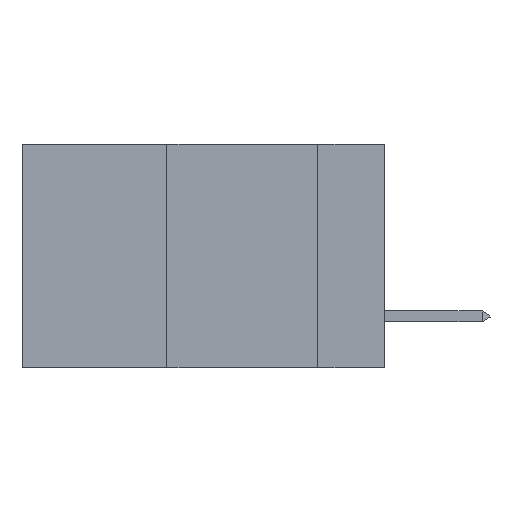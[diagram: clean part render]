
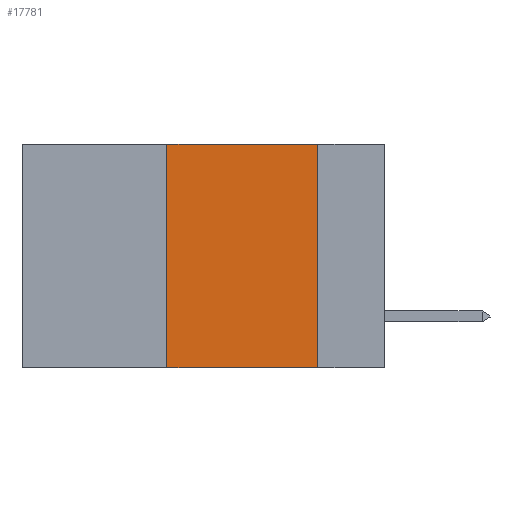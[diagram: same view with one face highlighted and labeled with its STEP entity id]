
A CAD part, left-side view. The second image highlights one B-rep face of the part: STEP entity #17781.
In plain terms, the highlighted planar face has unit normal (-1, 0, 0).
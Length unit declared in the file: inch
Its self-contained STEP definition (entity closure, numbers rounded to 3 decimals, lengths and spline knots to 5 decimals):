
#374 = VERTEX_POINT ( 'NONE', #19010 ) ;
#753 = LINE ( 'NONE', #11042, #24268 ) ;
#932 = EDGE_CURVE ( 'NONE', #9801, #8895, #753, .T. ) ;
#3188 = EDGE_CURVE ( 'NONE', #374, #9801, #9167, .T. ) ;
#3672 = ORIENTED_EDGE ( 'NONE', *, *, #3188, .F. ) ;
#4188 = PLANE ( 'NONE',  #22595 ) ;
#6211 = DIRECTION ( 'NONE',  ( 0., 0., -1. ) ) ;
#6673 = EDGE_CURVE ( 'NONE', #374, #9300, #23012, .T. ) ;
#7080 = VECTOR ( 'NONE', #19798, 39.37008 ) ;
#7840 = DIRECTION ( 'NONE',  ( 0., 0., -1. ) ) ;
#8378 = VECTOR ( 'NONE', #7840, 39.37008 ) ;
#8895 = VERTEX_POINT ( 'NONE', #22441 ) ;
#9167 = LINE ( 'NONE', #19589, #11698 ) ;
#9300 = VERTEX_POINT ( 'NONE', #22084 ) ;
#9801 = VERTEX_POINT ( 'NONE', #12863 ) ;
#11042 = CARTESIAN_POINT ( 'NONE',  ( 0., 0.6, 0. ) ) ;
#11698 = VECTOR ( 'NONE', #21257, 39.37008 ) ;
#11989 = EDGE_LOOP ( 'NONE', ( #22956, #21426, #3672, #14095 ) ) ;
#12863 = CARTESIAN_POINT ( 'NONE',  ( 0., 0.36, 0. ) ) ;
#14095 = ORIENTED_EDGE ( 'NONE', *, *, #6673, .T. ) ;
#15065 = LINE ( 'NONE', #15929, #8378 ) ;
#15274 = EDGE_CURVE ( 'NONE', #8895, #9300, #15065, .T. ) ;
#15917 = CARTESIAN_POINT ( 'NONE',  ( 0., 0.6, -0.37 ) ) ;
#15929 = CARTESIAN_POINT ( 'NONE',  ( 0., 0.11, 0. ) ) ;
#17781 = ADVANCED_FACE ( 'NONE', ( #20297 ), #4188, .F. ) ;
#18415 = CARTESIAN_POINT ( 'NONE',  ( 0., 0.6, 0. ) ) ;
#19010 = CARTESIAN_POINT ( 'NONE',  ( 0., 0.36, -0.37 ) ) ;
#19212 = DIRECTION ( 'NONE',  ( 0., -1., 0. ) ) ;
#19589 = CARTESIAN_POINT ( 'NONE',  ( 0., 0.36, 0. ) ) ;
#19798 = DIRECTION ( 'NONE',  ( 0., -1., 0. ) ) ;
#20297 = FACE_OUTER_BOUND ( 'NONE', #11989, .T. ) ;
#21257 = DIRECTION ( 'NONE',  ( 0., 0., 1. ) ) ;
#21426 = ORIENTED_EDGE ( 'NONE', *, *, #932, .F. ) ;
#22084 = CARTESIAN_POINT ( 'NONE',  ( 0., 0.11, -0.37 ) ) ;
#22441 = CARTESIAN_POINT ( 'NONE',  ( 0., 0.11, 0. ) ) ;
#22595 = AXIS2_PLACEMENT_3D ( 'NONE', #18415, #24285, #6211 ) ;
#22956 = ORIENTED_EDGE ( 'NONE', *, *, #15274, .F. ) ;
#23012 = LINE ( 'NONE', #15917, #7080 ) ;
#24268 = VECTOR ( 'NONE', #19212, 39.37008 ) ;
#24285 = DIRECTION ( 'NONE',  ( 1., 0., 0. ) ) ;
